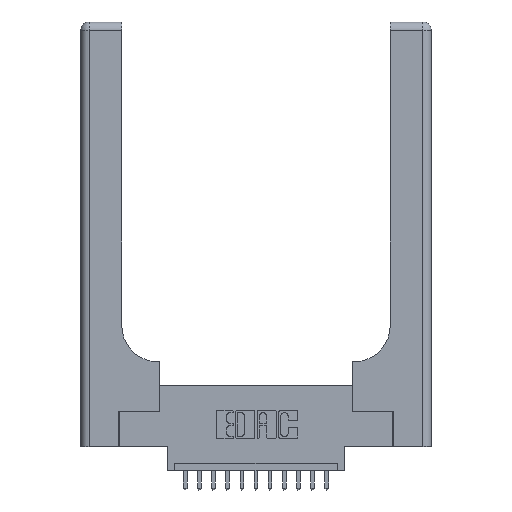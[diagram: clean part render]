
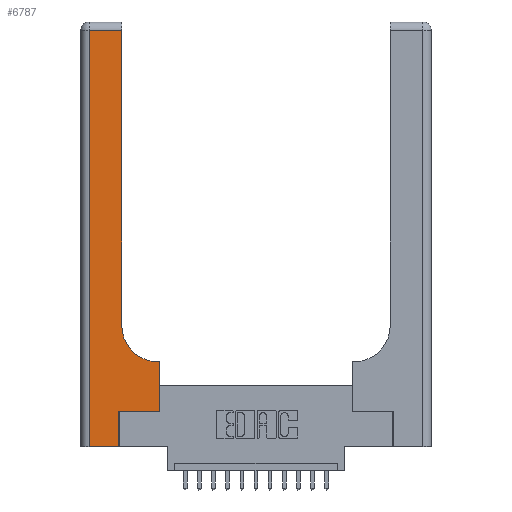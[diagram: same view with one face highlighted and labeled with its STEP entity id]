
A CAD part, top view. The second image highlights one B-rep face of the part: STEP entity #6787.
In plain terms, the highlighted planar face has unit normal (0, 0, 1).
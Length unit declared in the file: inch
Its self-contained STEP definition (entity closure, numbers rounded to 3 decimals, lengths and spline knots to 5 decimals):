
#451 = CARTESIAN_POINT ( 'NONE',  ( 0.5585, 0.6, 0.37 ) ) ;
#461 = ORIENTED_EDGE ( 'NONE', *, *, #2491, .T. ) ;
#659 = CARTESIAN_POINT ( 'NONE',  ( 0., 3., 0.37 ) ) ;
#1151 = VECTOR ( 'NONE', #10039, 39.37008 ) ;
#1432 = CARTESIAN_POINT ( 'NONE',  ( 0.5415, 0.6, 0.37 ) ) ;
#1610 = CARTESIAN_POINT ( 'NONE',  ( 0.269, 0.25, 0.37 ) ) ;
#1622 = ORIENTED_EDGE ( 'NONE', *, *, #17571, .T. ) ;
#1709 = LINE ( 'NONE', #5587, #15847 ) ;
#1933 = DIRECTION ( 'NONE',  ( -1., 0., 0. ) ) ;
#2001 = LINE ( 'NONE', #2107, #13822 ) ;
#2107 = CARTESIAN_POINT ( 'NONE',  ( 0.2915, 3., 0.37 ) ) ;
#2233 = VERTEX_POINT ( 'NONE', #14184 ) ;
#2253 = EDGE_CURVE ( 'NONE', #10151, #13192, #2001, .T. ) ;
#2491 = EDGE_CURVE ( 'NONE', #15012, #14318, #17666, .T. ) ;
#2619 = CARTESIAN_POINT ( 'NONE',  ( 0.269, 0.25, 0.37 ) ) ;
#3087 = ORIENTED_EDGE ( 'NONE', *, *, #6701, .T. ) ;
#4287 = VECTOR ( 'NONE', #16974, 39.37008 ) ;
#4510 = VECTOR ( 'NONE', #4930, 39.37008 ) ;
#4715 = CARTESIAN_POINT ( 'NONE',  ( 0., 2.94, 0.37 ) ) ;
#4743 = ORIENTED_EDGE ( 'NONE', *, *, #5387, .T. ) ;
#4745 = CARTESIAN_POINT ( 'NONE',  ( 0.269, 0., 0.37 ) ) ;
#4930 = DIRECTION ( 'NONE',  ( 0., 1., 0. ) ) ;
#5062 = ORIENTED_EDGE ( 'NONE', *, *, #17564, .T. ) ;
#5387 = EDGE_CURVE ( 'NONE', #14848, #8269, #17804, .T. ) ;
#5587 = CARTESIAN_POINT ( 'NONE',  ( 0.06, 3., 0.37 ) ) ;
#5931 = LINE ( 'NONE', #8091, #8111 ) ;
#6131 = PLANE ( 'NONE',  #7848 ) ;
#6175 = LINE ( 'NONE', #4715, #4287 ) ;
#6572 = ORIENTED_EDGE ( 'NONE', *, *, #6753, .T. ) ;
#6637 = EDGE_CURVE ( 'NONE', #2233, #15012, #1709, .T. ) ;
#6701 = EDGE_CURVE ( 'NONE', #14318, #7641, #8378, .T. ) ;
#6753 = EDGE_CURVE ( 'NONE', #14811, #10151, #16051, .T. ) ;
#6787 = ADVANCED_FACE ( 'NONE', ( #10976 ), #6131, .F. ) ;
#7144 = ORIENTED_EDGE ( 'NONE', *, *, #7300, .T. ) ;
#7182 = EDGE_LOOP ( 'NONE', ( #10997, #7144, #10247, #461, #3087, #5062, #4743, #1622, #6572 ) ) ;
#7300 = EDGE_CURVE ( 'NONE', #13192, #2233, #6175, .T. ) ;
#7393 = DIRECTION ( 'NONE',  ( 0., 1., 0. ) ) ;
#7630 = DIRECTION ( 'NONE',  ( 0., 1., 0. ) ) ;
#7641 = VERTEX_POINT ( 'NONE', #1610 ) ;
#7848 = AXIS2_PLACEMENT_3D ( 'NONE', #659, #14464, #1933 ) ;
#8091 = CARTESIAN_POINT ( 'NONE',  ( 0.2915, 0.6, 0.37 ) ) ;
#8111 = VECTOR ( 'NONE', #12298, 39.37008 ) ;
#8269 = VERTEX_POINT ( 'NONE', #451 ) ;
#8285 = CARTESIAN_POINT ( 'NONE',  ( 0.5585, 0.25, 0.37 ) ) ;
#8378 = LINE ( 'NONE', #4745, #4510 ) ;
#8536 = CARTESIAN_POINT ( 'NONE',  ( 0., 0., 0.37 ) ) ;
#10039 = DIRECTION ( 'NONE',  ( 1., 0., 0. ) ) ;
#10151 = VERTEX_POINT ( 'NONE', #16177 ) ;
#10247 = ORIENTED_EDGE ( 'NONE', *, *, #6637, .T. ) ;
#10856 = DIRECTION ( 'NONE',  ( 0., 0., -1. ) ) ;
#10976 = FACE_OUTER_BOUND ( 'NONE', #7182, .T. ) ;
#10997 = ORIENTED_EDGE ( 'NONE', *, *, #2253, .T. ) ;
#11056 = DIRECTION ( 'NONE',  ( 1., 0., 0. ) ) ;
#11143 = DIRECTION ( 'NONE',  ( 0., -1., 0. ) ) ;
#12298 = DIRECTION ( 'NONE',  ( -1., 0., 0. ) ) ;
#13119 = AXIS2_PLACEMENT_3D ( 'NONE', #13128, #10856, #15455 ) ;
#13128 = CARTESIAN_POINT ( 'NONE',  ( 0.5415, 0.85, 0.37 ) ) ;
#13192 = VERTEX_POINT ( 'NONE', #17617 ) ;
#13822 = VECTOR ( 'NONE', #7630, 39.37008 ) ;
#14108 = VECTOR ( 'NONE', #11056, 39.37008 ) ;
#14184 = CARTESIAN_POINT ( 'NONE',  ( 0.06, 2.94, 0.37 ) ) ;
#14318 = VERTEX_POINT ( 'NONE', #16359 ) ;
#14464 = DIRECTION ( 'NONE',  ( 0., 0., -1. ) ) ;
#14811 = VERTEX_POINT ( 'NONE', #1432 ) ;
#14848 = VERTEX_POINT ( 'NONE', #8285 ) ;
#15012 = VERTEX_POINT ( 'NONE', #16655 ) ;
#15225 = VECTOR ( 'NONE', #7393, 39.37008 ) ;
#15455 = DIRECTION ( 'NONE',  ( 1., 0., 0. ) ) ;
#15575 = CARTESIAN_POINT ( 'NONE',  ( 0.5585, 0.25, 0.37 ) ) ;
#15847 = VECTOR ( 'NONE', #11143, 39.37008 ) ;
#16051 = CIRCLE ( 'NONE', #13119, 0.25 ) ;
#16177 = CARTESIAN_POINT ( 'NONE',  ( 0.2915, 0.85, 0.37 ) ) ;
#16359 = CARTESIAN_POINT ( 'NONE',  ( 0.269, 0., 0.37 ) ) ;
#16655 = CARTESIAN_POINT ( 'NONE',  ( 0.06, 0., 0.37 ) ) ;
#16974 = DIRECTION ( 'NONE',  ( -1., 0., 0. ) ) ;
#17520 = LINE ( 'NONE', #2619, #14108 ) ;
#17564 = EDGE_CURVE ( 'NONE', #7641, #14848, #17520, .T. ) ;
#17571 = EDGE_CURVE ( 'NONE', #8269, #14811, #5931, .T. ) ;
#17617 = CARTESIAN_POINT ( 'NONE',  ( 0.2915, 2.94, 0.37 ) ) ;
#17666 = LINE ( 'NONE', #8536, #1151 ) ;
#17804 = LINE ( 'NONE', #15575, #15225 ) ;
